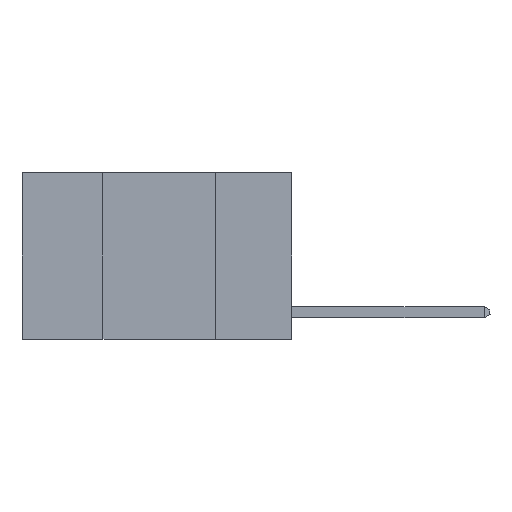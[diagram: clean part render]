
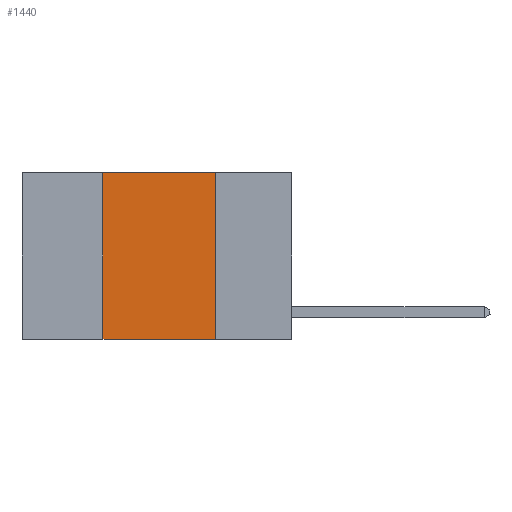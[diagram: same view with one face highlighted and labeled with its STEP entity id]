
A CAD part, left-side view. The second image highlights one B-rep face of the part: STEP entity #1440.
In plain terms, the highlighted planar face has unit normal (-1, 0, 0).
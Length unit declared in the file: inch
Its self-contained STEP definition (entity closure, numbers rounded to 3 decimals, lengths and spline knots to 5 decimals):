
#494 = CARTESIAN_POINT ( 'NONE',  ( 0., 0.6, 0. ) ) ;
#896 = EDGE_CURVE ( 'NONE', #9559, #14966, #8679, .T. ) ;
#1287 = AXIS2_PLACEMENT_3D ( 'NONE', #494, #1916, #10301 ) ;
#1419 = CARTESIAN_POINT ( 'NONE',  ( 0., 0.42, 0. ) ) ;
#1440 = ADVANCED_FACE ( 'NONE', ( #10511 ), #12479, .F. ) ;
#1480 = DIRECTION ( 'NONE',  ( 0., -1., 0. ) ) ;
#1916 = DIRECTION ( 'NONE',  ( 1., 0., 0. ) ) ;
#2575 = ORIENTED_EDGE ( 'NONE', *, *, #8173, .F. ) ;
#2850 = VERTEX_POINT ( 'NONE', #5470 ) ;
#3682 = LINE ( 'NONE', #16578, #5952 ) ;
#5470 = CARTESIAN_POINT ( 'NONE',  ( 0., 0.42, 0. ) ) ;
#5952 = VECTOR ( 'NONE', #1480, 39.37008 ) ;
#6012 = LINE ( 'NONE', #16052, #8011 ) ;
#8011 = VECTOR ( 'NONE', #21133, 39.37008 ) ;
#8173 = EDGE_CURVE ( 'NONE', #9559, #2850, #12870, .T. ) ;
#8460 = CARTESIAN_POINT ( 'NONE',  ( 0., 0.6, -0.37 ) ) ;
#8679 = LINE ( 'NONE', #8460, #19007 ) ;
#9559 = VERTEX_POINT ( 'NONE', #11870 ) ;
#9597 = CARTESIAN_POINT ( 'NONE',  ( 0., 0.17, 0. ) ) ;
#10107 = DIRECTION ( 'NONE',  ( 0., -1., 0. ) ) ;
#10301 = DIRECTION ( 'NONE',  ( 0., 0., -1. ) ) ;
#10511 = FACE_OUTER_BOUND ( 'NONE', #20225, .T. ) ;
#11395 = EDGE_CURVE ( 'NONE', #21495, #14966, #6012, .T. ) ;
#11870 = CARTESIAN_POINT ( 'NONE',  ( 0., 0.42, -0.37 ) ) ;
#12479 = PLANE ( 'NONE',  #1287 ) ;
#12703 = EDGE_CURVE ( 'NONE', #2850, #21495, #3682, .T. ) ;
#12870 = LINE ( 'NONE', #1419, #19225 ) ;
#12916 = ORIENTED_EDGE ( 'NONE', *, *, #11395, .F. ) ;
#13969 = CARTESIAN_POINT ( 'NONE',  ( 0., 0.17, -0.37 ) ) ;
#14966 = VERTEX_POINT ( 'NONE', #13969 ) ;
#16052 = CARTESIAN_POINT ( 'NONE',  ( 0., 0.17, 0. ) ) ;
#16578 = CARTESIAN_POINT ( 'NONE',  ( 0., 0.6, 0. ) ) ;
#19007 = VECTOR ( 'NONE', #10107, 39.37008 ) ;
#19225 = VECTOR ( 'NONE', #21295, 39.37008 ) ;
#20225 = EDGE_LOOP ( 'NONE', ( #12916, #21623, #2575, #20413 ) ) ;
#20413 = ORIENTED_EDGE ( 'NONE', *, *, #896, .T. ) ;
#21133 = DIRECTION ( 'NONE',  ( 0., 0., -1. ) ) ;
#21295 = DIRECTION ( 'NONE',  ( 0., 0., 1. ) ) ;
#21495 = VERTEX_POINT ( 'NONE', #9597 ) ;
#21623 = ORIENTED_EDGE ( 'NONE', *, *, #12703, .F. ) ;
